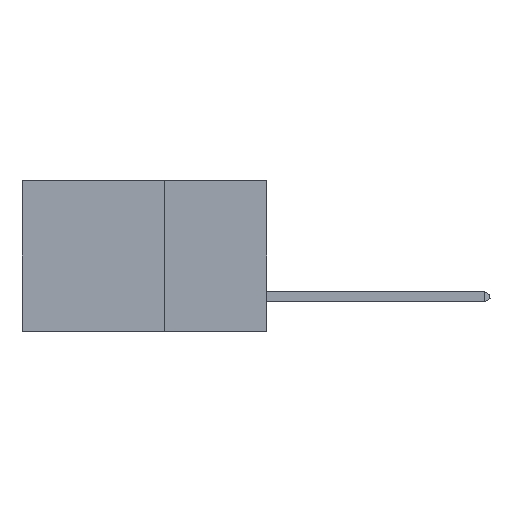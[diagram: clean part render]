
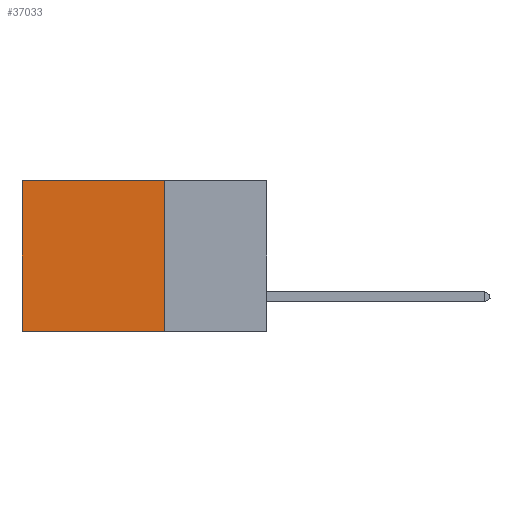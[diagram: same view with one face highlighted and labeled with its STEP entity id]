
A CAD part, left-side view. The second image highlights one B-rep face of the part: STEP entity #37033.
In plain terms, the highlighted planar face has unit normal (-1, 0, 0).
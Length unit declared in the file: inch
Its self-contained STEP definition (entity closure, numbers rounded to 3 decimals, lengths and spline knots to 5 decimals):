
#2528 = EDGE_CURVE ( 'NONE', #26915, #37321, #31220, .T. ) ;
#3216 = ORIENTED_EDGE ( 'NONE', *, *, #39268, .T. ) ;
#3273 = CARTESIAN_POINT ( 'NONE',  ( 0.2875, 0.25, 0. ) ) ;
#3932 = CARTESIAN_POINT ( 'NONE',  ( 0.2875, 0.6, 0. ) ) ;
#4334 = CARTESIAN_POINT ( 'NONE',  ( 0.2875, 0.25, 0. ) ) ;
#5986 = DIRECTION ( 'NONE',  ( 1., 0., 0. ) ) ;
#6098 = LINE ( 'NONE', #18971, #31886 ) ;
#6644 = VECTOR ( 'NONE', #19657, 39.37008 ) ;
#8372 = VECTOR ( 'NONE', #17713, 39.37008 ) ;
#8553 = EDGE_CURVE ( 'NONE', #36065, #10371, #12985, .T. ) ;
#8663 = VECTOR ( 'NONE', #38068, 39.37008 ) ;
#10371 = VERTEX_POINT ( 'NONE', #3932 ) ;
#10529 = ORIENTED_EDGE ( 'NONE', *, *, #8553, .T. ) ;
#11257 = AXIS2_PLACEMENT_3D ( 'NONE', #3273, #5986, #27747 ) ;
#11320 = CARTESIAN_POINT ( 'NONE',  ( 0.2875, 0.25, -0.37 ) ) ;
#12985 = LINE ( 'NONE', #4334, #8663 ) ;
#17713 = DIRECTION ( 'NONE',  ( 0., 1., 0. ) ) ;
#17948 = EDGE_LOOP ( 'NONE', ( #3216, #19736, #33948, #10529 ) ) ;
#18744 = PLANE ( 'NONE',  #11257 ) ;
#18971 = CARTESIAN_POINT ( 'NONE',  ( 0.2875, 0.25, 0. ) ) ;
#19657 = DIRECTION ( 'NONE',  ( 0., 0., -1. ) ) ;
#19736 = ORIENTED_EDGE ( 'NONE', *, *, #2528, .F. ) ;
#22665 = CARTESIAN_POINT ( 'NONE',  ( 0.2875, 0.6, -0.37 ) ) ;
#26313 = CARTESIAN_POINT ( 'NONE',  ( 0.2875, 0.25, 0. ) ) ;
#26915 = VERTEX_POINT ( 'NONE', #27023 ) ;
#27023 = CARTESIAN_POINT ( 'NONE',  ( 0.2875, 0.25, -0.37 ) ) ;
#27747 = DIRECTION ( 'NONE',  ( 0., 0., -1. ) ) ;
#28218 = DIRECTION ( 'NONE',  ( 0., 0., -1. ) ) ;
#28682 = FACE_OUTER_BOUND ( 'NONE', #17948, .T. ) ;
#29524 = LINE ( 'NONE', #38313, #6644 ) ;
#31220 = LINE ( 'NONE', #11320, #8372 ) ;
#31886 = VECTOR ( 'NONE', #28218, 39.37008 ) ;
#33948 = ORIENTED_EDGE ( 'NONE', *, *, #34754, .F. ) ;
#34754 = EDGE_CURVE ( 'NONE', #36065, #26915, #6098, .T. ) ;
#36065 = VERTEX_POINT ( 'NONE', #26313 ) ;
#37033 = ADVANCED_FACE ( 'NONE', ( #28682 ), #18744, .F. ) ;
#37321 = VERTEX_POINT ( 'NONE', #22665 ) ;
#38068 = DIRECTION ( 'NONE',  ( 0., 1., 0. ) ) ;
#38313 = CARTESIAN_POINT ( 'NONE',  ( 0.2875, 0.6, 0. ) ) ;
#39268 = EDGE_CURVE ( 'NONE', #10371, #37321, #29524, .T. ) ;
